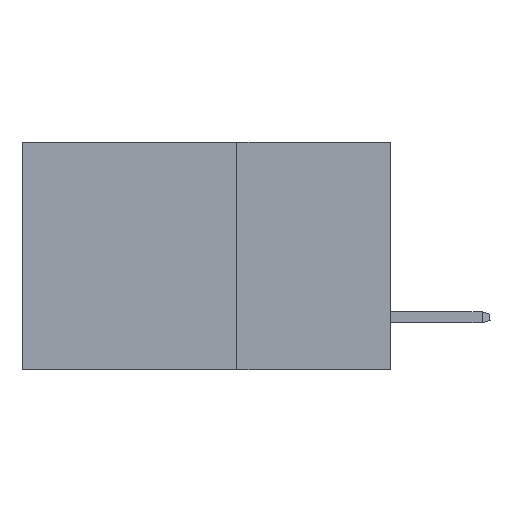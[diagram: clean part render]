
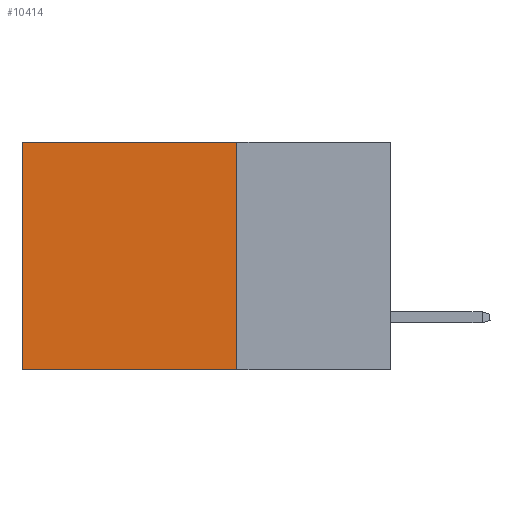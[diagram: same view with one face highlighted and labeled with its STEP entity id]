
A CAD part, left-side view. The second image highlights one B-rep face of the part: STEP entity #10414.
In plain terms, the highlighted planar face has unit normal (-1, 0, 0).
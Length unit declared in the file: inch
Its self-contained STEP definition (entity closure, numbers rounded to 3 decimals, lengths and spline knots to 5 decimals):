
#358 = EDGE_CURVE ( 'NONE', #24659, #13940, #18026, .T. ) ;
#454 = CARTESIAN_POINT ( 'NONE',  ( 0.2875, 0.25, 0. ) ) ;
#609 = ORIENTED_EDGE ( 'NONE', *, *, #9407, .T. ) ;
#3121 = DIRECTION ( 'NONE',  ( 0., 1., 0. ) ) ;
#4275 = FACE_OUTER_BOUND ( 'NONE', #29797, .T. ) ;
#4320 = CARTESIAN_POINT ( 'NONE',  ( 0.2875, 0.6, -0.37 ) ) ;
#5735 = CARTESIAN_POINT ( 'NONE',  ( 0.2875, 0.25, 0. ) ) ;
#6664 = CARTESIAN_POINT ( 'NONE',  ( 0.2875, 0.25, 0. ) ) ;
#9407 = EDGE_CURVE ( 'NONE', #24659, #32284, #9762, .T. ) ;
#9695 = VECTOR ( 'NONE', #27425, 39.37008 ) ;
#9762 = LINE ( 'NONE', #6664, #14151 ) ;
#10209 = EDGE_CURVE ( 'NONE', #13940, #31479, #13046, .T. ) ;
#10402 = DIRECTION ( 'NONE',  ( 0., 0., -1. ) ) ;
#10414 = ADVANCED_FACE ( 'NONE', ( #4275 ), #15840, .F. ) ;
#12333 = CARTESIAN_POINT ( 'NONE',  ( 0.2875, 0.25, -0.37 ) ) ;
#12606 = VECTOR ( 'NONE', #34955, 39.37008 ) ;
#13046 = LINE ( 'NONE', #25696, #12606 ) ;
#13940 = VERTEX_POINT ( 'NONE', #12333 ) ;
#14151 = VECTOR ( 'NONE', #3121, 39.37008 ) ;
#14444 = LINE ( 'NONE', #26004, #22227 ) ;
#15840 = PLANE ( 'NONE',  #18058 ) ;
#17961 = ORIENTED_EDGE ( 'NONE', *, *, #29943, .T. ) ;
#18026 = LINE ( 'NONE', #5735, #9695 ) ;
#18058 = AXIS2_PLACEMENT_3D ( 'NONE', #454, #38325, #10402 ) ;
#19321 = DIRECTION ( 'NONE',  ( 0., 0., -1. ) ) ;
#22227 = VECTOR ( 'NONE', #19321, 39.37008 ) ;
#23744 = CARTESIAN_POINT ( 'NONE',  ( 0.2875, 0.25, 0. ) ) ;
#24659 = VERTEX_POINT ( 'NONE', #23744 ) ;
#25696 = CARTESIAN_POINT ( 'NONE',  ( 0.2875, 0.25, -0.37 ) ) ;
#26004 = CARTESIAN_POINT ( 'NONE',  ( 0.2875, 0.6, 0. ) ) ;
#27425 = DIRECTION ( 'NONE',  ( 0., 0., -1. ) ) ;
#27889 = ORIENTED_EDGE ( 'NONE', *, *, #10209, .F. ) ;
#29797 = EDGE_LOOP ( 'NONE', ( #17961, #27889, #30131, #609 ) ) ;
#29943 = EDGE_CURVE ( 'NONE', #32284, #31479, #14444, .T. ) ;
#30131 = ORIENTED_EDGE ( 'NONE', *, *, #358, .F. ) ;
#31479 = VERTEX_POINT ( 'NONE', #4320 ) ;
#32284 = VERTEX_POINT ( 'NONE', #36728 ) ;
#34955 = DIRECTION ( 'NONE',  ( 0., 1., 0. ) ) ;
#36728 = CARTESIAN_POINT ( 'NONE',  ( 0.2875, 0.6, 0. ) ) ;
#38325 = DIRECTION ( 'NONE',  ( 1., 0., 0. ) ) ;
